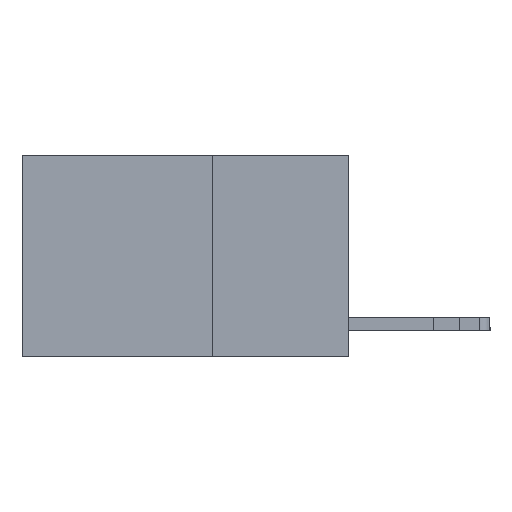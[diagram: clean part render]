
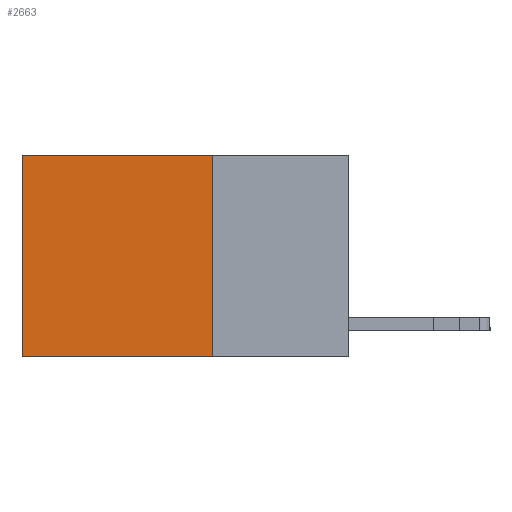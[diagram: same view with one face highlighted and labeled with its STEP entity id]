
A CAD part, left-side view. The second image highlights one B-rep face of the part: STEP entity #2663.
In plain terms, the highlighted planar face has unit normal (-1, 0, 0).
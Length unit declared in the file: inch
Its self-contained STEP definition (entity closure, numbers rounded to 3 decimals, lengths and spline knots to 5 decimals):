
#283 = CARTESIAN_POINT ( 'NONE',  ( 0.2625, 0.6, 0. ) ) ;
#302 = CARTESIAN_POINT ( 'NONE',  ( 0.2625, 0.25, 0. ) ) ;
#804 = CARTESIAN_POINT ( 'NONE',  ( 0.2625, 0.6, 0. ) ) ;
#871 = DIRECTION ( 'NONE',  ( 0., 1., 0. ) ) ;
#1199 = LINE ( 'NONE', #15030, #2197 ) ;
#1917 = VECTOR ( 'NONE', #871, 39.37008 ) ;
#2197 = VECTOR ( 'NONE', #7409, 39.37008 ) ;
#2663 = ADVANCED_FACE ( 'NONE', ( #10283 ), #14057, .F. ) ;
#3281 = VERTEX_POINT ( 'NONE', #11045 ) ;
#3453 = VECTOR ( 'NONE', #12261, 39.37008 ) ;
#3684 = EDGE_CURVE ( 'NONE', #10236, #9616, #16119, .T. ) ;
#3789 = EDGE_LOOP ( 'NONE', ( #4091, #5768, #14746, #15465 ) ) ;
#4091 = ORIENTED_EDGE ( 'NONE', *, *, #3684, .T. ) ;
#4709 = VECTOR ( 'NONE', #15272, 39.37008 ) ;
#5768 = ORIENTED_EDGE ( 'NONE', *, *, #10047, .F. ) ;
#7409 = DIRECTION ( 'NONE',  ( 0., 0., -1. ) ) ;
#7802 = CARTESIAN_POINT ( 'NONE',  ( 0.2625, 0.25, -0.37 ) ) ;
#9616 = VERTEX_POINT ( 'NONE', #13572 ) ;
#9644 = VERTEX_POINT ( 'NONE', #302 ) ;
#9783 = LINE ( 'NONE', #12170, #1917 ) ;
#10047 = EDGE_CURVE ( 'NONE', #3281, #9616, #11338, .T. ) ;
#10236 = VERTEX_POINT ( 'NONE', #283 ) ;
#10283 = FACE_OUTER_BOUND ( 'NONE', #3789, .T. ) ;
#11045 = CARTESIAN_POINT ( 'NONE',  ( 0.2625, 0.25, -0.37 ) ) ;
#11338 = LINE ( 'NONE', #7802, #4709 ) ;
#11522 = CARTESIAN_POINT ( 'NONE',  ( 0.2625, 0.25, 0. ) ) ;
#12170 = CARTESIAN_POINT ( 'NONE',  ( 0.2625, 0.25, 0. ) ) ;
#12261 = DIRECTION ( 'NONE',  ( 0., 0., -1. ) ) ;
#13572 = CARTESIAN_POINT ( 'NONE',  ( 0.2625, 0.6, -0.37 ) ) ;
#14057 = PLANE ( 'NONE',  #14108 ) ;
#14108 = AXIS2_PLACEMENT_3D ( 'NONE', #11522, #15217, #15296 ) ;
#14746 = ORIENTED_EDGE ( 'NONE', *, *, #15177, .F. ) ;
#15030 = CARTESIAN_POINT ( 'NONE',  ( 0.2625, 0.25, 0. ) ) ;
#15067 = EDGE_CURVE ( 'NONE', #9644, #10236, #9783, .T. ) ;
#15177 = EDGE_CURVE ( 'NONE', #9644, #3281, #1199, .T. ) ;
#15217 = DIRECTION ( 'NONE',  ( 1., 0., 0. ) ) ;
#15272 = DIRECTION ( 'NONE',  ( 0., 1., 0. ) ) ;
#15296 = DIRECTION ( 'NONE',  ( 0., 0., -1. ) ) ;
#15465 = ORIENTED_EDGE ( 'NONE', *, *, #15067, .T. ) ;
#16119 = LINE ( 'NONE', #804, #3453 ) ;
